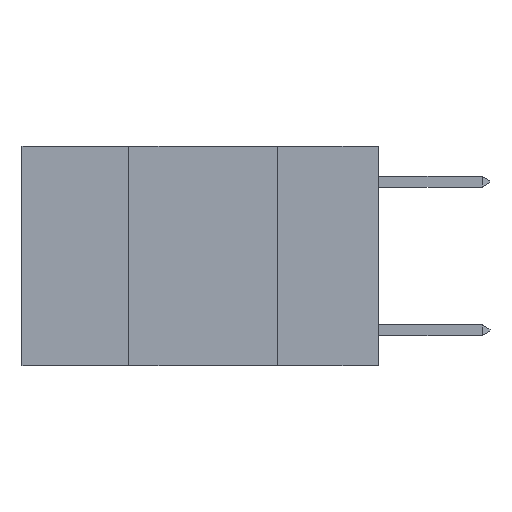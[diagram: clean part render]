
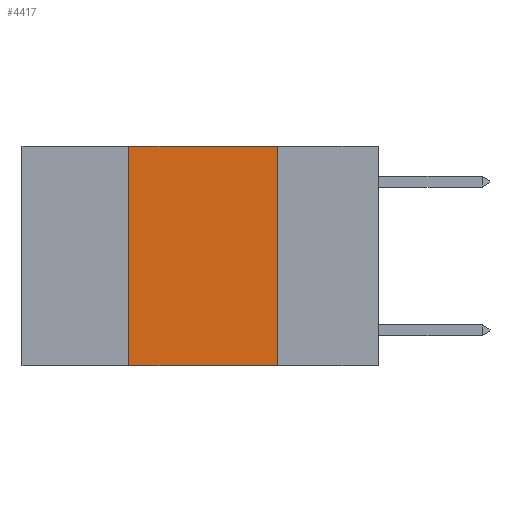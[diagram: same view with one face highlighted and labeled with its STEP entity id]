
A CAD part, left-side view. The second image highlights one B-rep face of the part: STEP entity #4417.
In plain terms, the highlighted planar face has unit normal (-1, 0, 0).
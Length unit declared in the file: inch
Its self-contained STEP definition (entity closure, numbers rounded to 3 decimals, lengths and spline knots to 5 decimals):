
#196 = EDGE_CURVE ( 'NONE', #3561, #4617, #9091, .T. ) ;
#987 = CARTESIAN_POINT ( 'NONE',  ( 0., 0.6, 0. ) ) ;
#1028 = ORIENTED_EDGE ( 'NONE', *, *, #10521, .T. ) ;
#1334 = ORIENTED_EDGE ( 'NONE', *, *, #4333, .F. ) ;
#1971 = DIRECTION ( 'NONE',  ( 0., -1., 0. ) ) ;
#2087 = DIRECTION ( 'NONE',  ( 1., 0., 0. ) ) ;
#2218 = AXIS2_PLACEMENT_3D ( 'NONE', #7728, #2087, #8663 ) ;
#2221 = CARTESIAN_POINT ( 'NONE',  ( 0., 0.17, 0. ) ) ;
#2328 = DIRECTION ( 'NONE',  ( 0., 0., -1. ) ) ;
#2920 = VERTEX_POINT ( 'NONE', #2221 ) ;
#3231 = CARTESIAN_POINT ( 'NONE',  ( 0., 0.42, -0.37 ) ) ;
#3291 = CARTESIAN_POINT ( 'NONE',  ( 0., 0.42, 0. ) ) ;
#3561 = VERTEX_POINT ( 'NONE', #3231 ) ;
#4079 = EDGE_CURVE ( 'NONE', #2920, #4198, #8283, .T. ) ;
#4198 = VERTEX_POINT ( 'NONE', #5374 ) ;
#4333 = EDGE_CURVE ( 'NONE', #4617, #2920, #10493, .T. ) ;
#4417 = ADVANCED_FACE ( 'NONE', ( #6606 ), #10467, .F. ) ;
#4617 = VERTEX_POINT ( 'NONE', #3291 ) ;
#5374 = CARTESIAN_POINT ( 'NONE',  ( 0., 0.17, -0.37 ) ) ;
#5806 = VECTOR ( 'NONE', #2328, 39.37008 ) ;
#5877 = CARTESIAN_POINT ( 'NONE',  ( 0., 0.42, 0. ) ) ;
#6606 = FACE_OUTER_BOUND ( 'NONE', #6729, .T. ) ;
#6729 = EDGE_LOOP ( 'NONE', ( #9569, #1334, #9178, #1028 ) ) ;
#7728 = CARTESIAN_POINT ( 'NONE',  ( 0., 0.6, 0. ) ) ;
#8094 = CARTESIAN_POINT ( 'NONE',  ( 0., 0.6, -0.37 ) ) ;
#8283 = LINE ( 'NONE', #8912, #5806 ) ;
#8663 = DIRECTION ( 'NONE',  ( 0., 0., -1. ) ) ;
#8912 = CARTESIAN_POINT ( 'NONE',  ( 0., 0.17, 0. ) ) ;
#9028 = DIRECTION ( 'NONE',  ( 0., -1., 0. ) ) ;
#9091 = LINE ( 'NONE', #5877, #11483 ) ;
#9178 = ORIENTED_EDGE ( 'NONE', *, *, #196, .F. ) ;
#9384 = LINE ( 'NONE', #8094, #11218 ) ;
#9569 = ORIENTED_EDGE ( 'NONE', *, *, #4079, .F. ) ;
#10214 = VECTOR ( 'NONE', #1971, 39.37008 ) ;
#10467 = PLANE ( 'NONE',  #2218 ) ;
#10493 = LINE ( 'NONE', #987, #10214 ) ;
#10521 = EDGE_CURVE ( 'NONE', #3561, #4198, #9384, .T. ) ;
#11158 = DIRECTION ( 'NONE',  ( 0., 0., 1. ) ) ;
#11218 = VECTOR ( 'NONE', #9028, 39.37008 ) ;
#11483 = VECTOR ( 'NONE', #11158, 39.37008 ) ;
